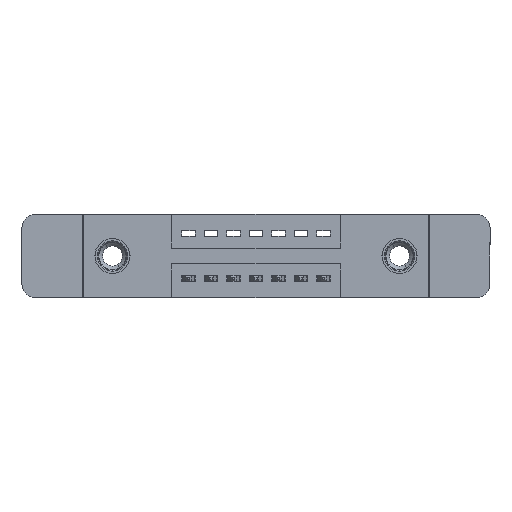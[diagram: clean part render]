
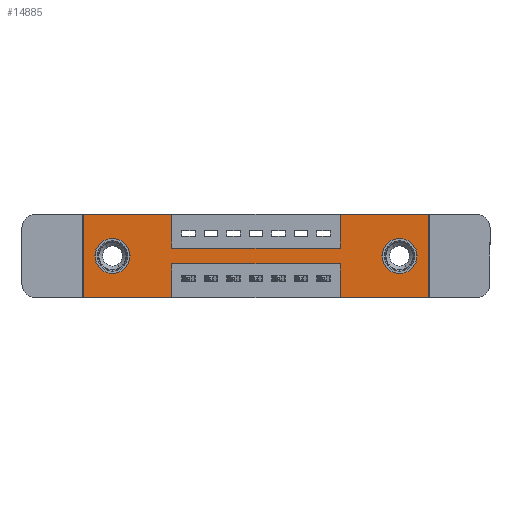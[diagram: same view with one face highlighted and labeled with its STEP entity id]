
A CAD part, front view. The second image highlights one B-rep face of the part: STEP entity #14885.
In plain terms, the highlighted planar face has unit normal (0, -1, 0).
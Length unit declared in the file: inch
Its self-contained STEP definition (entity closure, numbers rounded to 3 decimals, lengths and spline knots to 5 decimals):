
#182 = CARTESIAN_POINT ( 'NONE',  ( 1.535, 0., -0.37 ) ) ;
#278 = CARTESIAN_POINT ( 'NONE',  ( 0.3925, 0., -0.37 ) ) ;
#279 = ORIENTED_EDGE ( 'NONE', *, *, #499, .F. ) ;
#462 = ORIENTED_EDGE ( 'NONE', *, *, #10651, .F. ) ;
#476 = CARTESIAN_POINT ( 'NONE',  ( 1.1425, 0., -0.37 ) ) ;
#499 = EDGE_CURVE ( 'NONE', #12639, #2811, #1391, .T. ) ;
#832 = ORIENTED_EDGE ( 'NONE', *, *, #13940, .F. ) ;
#873 = DIRECTION ( 'NONE',  ( 0., 1., 0. ) ) ;
#941 = CARTESIAN_POINT ( 'NONE',  ( 0., 0., -0.37 ) ) ;
#950 = EDGE_CURVE ( 'NONE', #4221, #12639, #5558, .T. ) ;
#984 = CARTESIAN_POINT ( 'NONE',  ( 0., 0., -0.37 ) ) ;
#1119 = LINE ( 'NONE', #984, #14471 ) ;
#1239 = DIRECTION ( 'NONE',  ( 1., 0., 0. ) ) ;
#1391 = LINE ( 'NONE', #14212, #12732 ) ;
#1521 = EDGE_CURVE ( 'NONE', #12126, #3258, #3532, .T. ) ;
#1557 = PLANE ( 'NONE',  #13157 ) ;
#1558 = CIRCLE ( 'NONE', #6354, 0.078 ) ;
#1687 = CIRCLE ( 'NONE', #10221, 0.078 ) ;
#1736 = VECTOR ( 'NONE', #8385, 39.37008 ) ;
#2042 = ORIENTED_EDGE ( 'NONE', *, *, #7419, .F. ) ;
#2170 = CARTESIAN_POINT ( 'NONE',  ( 1.405, 0., -0.263 ) ) ;
#2309 = EDGE_CURVE ( 'NONE', #3550, #10025, #9605, .T. ) ;
#2680 = DIRECTION ( 'NONE',  ( 0., 0., -1. ) ) ;
#2811 = VERTEX_POINT ( 'NONE', #12339 ) ;
#3232 = ORIENTED_EDGE ( 'NONE', *, *, #950, .F. ) ;
#3258 = VERTEX_POINT ( 'NONE', #2170 ) ;
#3329 = ORIENTED_EDGE ( 'NONE', *, *, #15009, .F. ) ;
#3523 = CARTESIAN_POINT ( 'NONE',  ( 0.3925, 0., 0. ) ) ;
#3532 = CIRCLE ( 'NONE', #14034, 0.078 ) ;
#3550 = VERTEX_POINT ( 'NONE', #10780 ) ;
#3708 = CARTESIAN_POINT ( 'NONE',  ( 1.535, 0., 0. ) ) ;
#3742 = LINE ( 'NONE', #11718, #8509 ) ;
#3763 = DIRECTION ( 'NONE',  ( 0., 1., 0. ) ) ;
#3866 = CARTESIAN_POINT ( 'NONE',  ( 0.3925, 0., 0. ) ) ;
#4071 = VECTOR ( 'NONE', #11316, 39.37008 ) ;
#4121 = CARTESIAN_POINT ( 'NONE',  ( 0.3925, 0., -0.15 ) ) ;
#4181 = EDGE_CURVE ( 'NONE', #10025, #14834, #13002, .T. ) ;
#4221 = VERTEX_POINT ( 'NONE', #278 ) ;
#4333 = VERTEX_POINT ( 'NONE', #476 ) ;
#4408 = CARTESIAN_POINT ( 'NONE',  ( 1.1425, 0., 0. ) ) ;
#4451 = CARTESIAN_POINT ( 'NONE',  ( 1.405, 0., -0.185 ) ) ;
#4765 = VERTEX_POINT ( 'NONE', #12853 ) ;
#4881 = CARTESIAN_POINT ( 'NONE',  ( 0.13, 0., -0.185 ) ) ;
#5305 = VERTEX_POINT ( 'NONE', #14937 ) ;
#5341 = FACE_BOUND ( 'NONE', #5835, .T. ) ;
#5455 = EDGE_CURVE ( 'NONE', #2811, #13327, #3742, .T. ) ;
#5543 = DIRECTION ( 'NONE',  ( 0., 1., 0. ) ) ;
#5550 = LINE ( 'NONE', #9473, #12891 ) ;
#5552 = CARTESIAN_POINT ( 'NONE',  ( 0., 0., 0. ) ) ;
#5558 = LINE ( 'NONE', #9289, #11615 ) ;
#5703 = DIRECTION ( 'NONE',  ( 0., 0., -1. ) ) ;
#5739 = CARTESIAN_POINT ( 'NONE',  ( 1.535, 0., 0. ) ) ;
#5835 = EDGE_LOOP ( 'NONE', ( #7863, #8835 ) ) ;
#5849 = VECTOR ( 'NONE', #12877, 39.37008 ) ;
#5865 = ORIENTED_EDGE ( 'NONE', *, *, #1521, .T. ) ;
#5980 = EDGE_CURVE ( 'NONE', #4333, #4765, #14878, .T. ) ;
#6104 = DIRECTION ( 'NONE',  ( 0., -1., 0. ) ) ;
#6317 = LINE ( 'NONE', #3866, #1736 ) ;
#6354 = AXIS2_PLACEMENT_3D ( 'NONE', #14433, #10849, #7412 ) ;
#6396 = DIRECTION ( 'NONE',  ( -1., 0., 0. ) ) ;
#6827 = ORIENTED_EDGE ( 'NONE', *, *, #2309, .F. ) ;
#7113 = ORIENTED_EDGE ( 'NONE', *, *, #5980, .F. ) ;
#7158 = CARTESIAN_POINT ( 'NONE',  ( 0.3925, 0., -0.15 ) ) ;
#7160 = VERTEX_POINT ( 'NONE', #4121 ) ;
#7198 = LINE ( 'NONE', #4408, #9042 ) ;
#7412 = DIRECTION ( 'NONE',  ( 0., 0., -1. ) ) ;
#7419 = EDGE_CURVE ( 'NONE', #14834, #4333, #1119, .T. ) ;
#7721 = FACE_BOUND ( 'NONE', #10821, .T. ) ;
#7810 = CARTESIAN_POINT ( 'NONE',  ( 1.405, 0., -0.107 ) ) ;
#7863 = ORIENTED_EDGE ( 'NONE', *, *, #8704, .T. ) ;
#7865 = EDGE_CURVE ( 'NONE', #7160, #7892, #14638, .T. ) ;
#7892 = VERTEX_POINT ( 'NONE', #9499 ) ;
#7927 = CARTESIAN_POINT ( 'NONE',  ( 1.1425, 0., -0.37 ) ) ;
#8084 = VECTOR ( 'NONE', #6396, 39.37008 ) ;
#8221 = DIRECTION ( 'NONE',  ( -1., 0., 0. ) ) ;
#8385 = DIRECTION ( 'NONE',  ( 0., 0., -1. ) ) ;
#8509 = VECTOR ( 'NONE', #1239, 39.37008 ) ;
#8704 = EDGE_CURVE ( 'NONE', #14413, #10214, #12991, .T. ) ;
#8835 = ORIENTED_EDGE ( 'NONE', *, *, #12349, .T. ) ;
#9016 = DIRECTION ( 'NONE',  ( 1., 0., 0. ) ) ;
#9042 = VECTOR ( 'NONE', #11322, 39.37008 ) ;
#9289 = CARTESIAN_POINT ( 'NONE',  ( 0., 0., -0.37 ) ) ;
#9473 = CARTESIAN_POINT ( 'NONE',  ( 0.3925, 0., -0.37 ) ) ;
#9499 = CARTESIAN_POINT ( 'NONE',  ( 1.1425, 0., -0.15 ) ) ;
#9605 = LINE ( 'NONE', #5552, #4071 ) ;
#9889 = AXIS2_PLACEMENT_3D ( 'NONE', #13706, #873, #14733 ) ;
#10025 = VERTEX_POINT ( 'NONE', #5739 ) ;
#10214 = VERTEX_POINT ( 'NONE', #13149 ) ;
#10221 = AXIS2_PLACEMENT_3D ( 'NONE', #4881, #3763, #10733 ) ;
#10283 = ORIENTED_EDGE ( 'NONE', *, *, #5455, .F. ) ;
#10298 = VECTOR ( 'NONE', #12536, 39.37008 ) ;
#10651 = EDGE_CURVE ( 'NONE', #13327, #7160, #6317, .T. ) ;
#10659 = LINE ( 'NONE', #14656, #8084 ) ;
#10671 = DIRECTION ( 'NONE',  ( 0., 0., 1. ) ) ;
#10733 = DIRECTION ( 'NONE',  ( 0., 0., 1. ) ) ;
#10780 = CARTESIAN_POINT ( 'NONE',  ( 1.1425, 0., 0. ) ) ;
#10816 = ORIENTED_EDGE ( 'NONE', *, *, #4181, .F. ) ;
#10821 = EDGE_LOOP ( 'NONE', ( #5865, #13203 ) ) ;
#10849 = DIRECTION ( 'NONE',  ( 0., 1., 0. ) ) ;
#11086 = EDGE_CURVE ( 'NONE', #3258, #12126, #1558, .T. ) ;
#11163 = ORIENTED_EDGE ( 'NONE', *, *, #7865, .F. ) ;
#11316 = DIRECTION ( 'NONE',  ( 1., 0., 0. ) ) ;
#11322 = DIRECTION ( 'NONE',  ( 0., 0., 1. ) ) ;
#11615 = VECTOR ( 'NONE', #8221, 39.37008 ) ;
#11718 = CARTESIAN_POINT ( 'NONE',  ( 0., 0., 0. ) ) ;
#11968 = CARTESIAN_POINT ( 'NONE',  ( 0., 0., -0.37 ) ) ;
#12126 = VERTEX_POINT ( 'NONE', #7810 ) ;
#12339 = CARTESIAN_POINT ( 'NONE',  ( 0., 0., 0. ) ) ;
#12349 = EDGE_CURVE ( 'NONE', #10214, #14413, #1687, .T. ) ;
#12536 = DIRECTION ( 'NONE',  ( 0., 0., 1. ) ) ;
#12639 = VERTEX_POINT ( 'NONE', #941 ) ;
#12732 = VECTOR ( 'NONE', #10671, 39.37008 ) ;
#12750 = ORIENTED_EDGE ( 'NONE', *, *, #14016, .F. ) ;
#12853 = CARTESIAN_POINT ( 'NONE',  ( 1.1425, 0., -0.22 ) ) ;
#12877 = DIRECTION ( 'NONE',  ( 0., 0., -1. ) ) ;
#12891 = VECTOR ( 'NONE', #5703, 39.37008 ) ;
#12991 = CIRCLE ( 'NONE', #9889, 0.078 ) ;
#13002 = LINE ( 'NONE', #3708, #5849 ) ;
#13149 = CARTESIAN_POINT ( 'NONE',  ( 0.13, 0., -0.263 ) ) ;
#13157 = AXIS2_PLACEMENT_3D ( 'NONE', #11968, #6104, #2680 ) ;
#13203 = ORIENTED_EDGE ( 'NONE', *, *, #11086, .T. ) ;
#13327 = VERTEX_POINT ( 'NONE', #3523 ) ;
#13573 = FACE_OUTER_BOUND ( 'NONE', #15034, .T. ) ;
#13705 = VECTOR ( 'NONE', #9016, 39.37008 ) ;
#13706 = CARTESIAN_POINT ( 'NONE',  ( 0.13, 0., -0.185 ) ) ;
#13940 = EDGE_CURVE ( 'NONE', #7892, #3550, #7198, .T. ) ;
#14016 = EDGE_CURVE ( 'NONE', #5305, #4221, #5550, .T. ) ;
#14034 = AXIS2_PLACEMENT_3D ( 'NONE', #4451, #5543, #15129 ) ;
#14212 = CARTESIAN_POINT ( 'NONE',  ( 0., 0., 0. ) ) ;
#14413 = VERTEX_POINT ( 'NONE', #14594 ) ;
#14433 = CARTESIAN_POINT ( 'NONE',  ( 1.405, 0., -0.185 ) ) ;
#14471 = VECTOR ( 'NONE', #15161, 39.37008 ) ;
#14594 = CARTESIAN_POINT ( 'NONE',  ( 0.13, 0., -0.107 ) ) ;
#14638 = LINE ( 'NONE', #7158, #13705 ) ;
#14656 = CARTESIAN_POINT ( 'NONE',  ( 0.3925, 0., -0.22 ) ) ;
#14733 = DIRECTION ( 'NONE',  ( 0., 0., 1. ) ) ;
#14834 = VERTEX_POINT ( 'NONE', #182 ) ;
#14878 = LINE ( 'NONE', #7927, #10298 ) ;
#14885 = ADVANCED_FACE ( 'NONE', ( #7721, #5341, #13573 ), #1557, .T. ) ;
#14937 = CARTESIAN_POINT ( 'NONE',  ( 0.3925, 0., -0.22 ) ) ;
#15009 = EDGE_CURVE ( 'NONE', #4765, #5305, #10659, .T. ) ;
#15034 = EDGE_LOOP ( 'NONE', ( #12750, #3329, #7113, #2042, #10816, #6827, #832, #11163, #462, #10283, #279, #3232 ) ) ;
#15129 = DIRECTION ( 'NONE',  ( 0., 0., -1. ) ) ;
#15161 = DIRECTION ( 'NONE',  ( -1., 0., 0. ) ) ;
